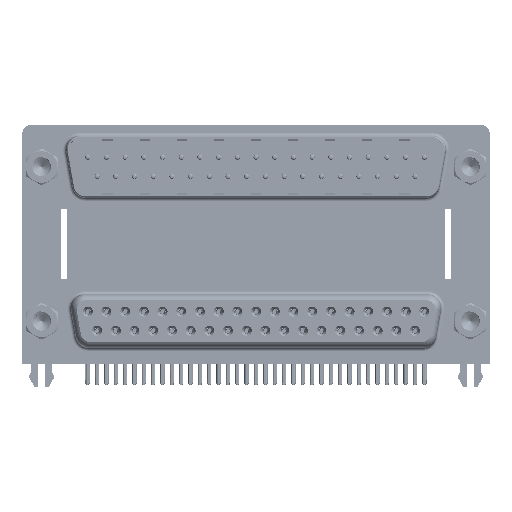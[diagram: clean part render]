
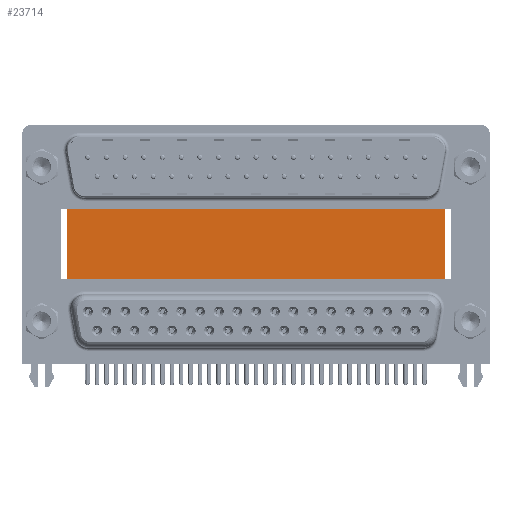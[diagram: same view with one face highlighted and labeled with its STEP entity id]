
A CAD part, top view. The second image highlights one B-rep face of the part: STEP entity #23714.
In plain terms, the highlighted planar face has unit normal (0, 0, 1).
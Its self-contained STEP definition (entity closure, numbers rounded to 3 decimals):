
#1918 = EDGE_CURVE ( 'NONE', #43277, #64732, #73841, .T. ) ;
#3527 = CARTESIAN_POINT ( 'NONE',  ( 3.79, 16.585, -12. ) ) ;
#3549 = CARTESIAN_POINT ( 'NONE',  ( 59.71, 16.585, -12. ) ) ;
#8940 = VERTEX_POINT ( 'NONE', #35187 ) ;
#10958 = ORIENTED_EDGE ( 'NONE', *, *, #48149, .F. ) ;
#12147 = ORIENTED_EDGE ( 'NONE', *, *, #1918, .F. ) ;
#13988 = LINE ( 'NONE', #25743, #72614 ) ;
#17152 = CARTESIAN_POINT ( 'NONE',  ( 59.71, 16.585, -12. ) ) ;
#21014 = DIRECTION ( 'NONE',  ( -1., 0., 0. ) ) ;
#23714 = ADVANCED_FACE ( 'NONE', ( #49443 ), #66976, .F. ) ;
#24715 = CARTESIAN_POINT ( 'NONE',  ( 3.79, -3.735, -12. ) ) ;
#25743 = CARTESIAN_POINT ( 'NONE',  ( 3.79, 16.585, -12. ) ) ;
#26696 = DIRECTION ( 'NONE',  ( 0., 0., -1. ) ) ;
#26873 = CARTESIAN_POINT ( 'NONE',  ( 59.71, -3.735, -12. ) ) ;
#29584 = EDGE_LOOP ( 'NONE', ( #45583, #12147, #10958, #63220 ) ) ;
#30680 = DIRECTION ( 'NONE',  ( 0., -1., 0. ) ) ;
#31212 = CARTESIAN_POINT ( 'NONE',  ( 3.79, 16.585, -12. ) ) ;
#34984 = VECTOR ( 'NONE', #59253, 1000. ) ;
#35187 = CARTESIAN_POINT ( 'NONE',  ( 3.79, 16.585, -12. ) ) ;
#35402 = LINE ( 'NONE', #31212, #56946 ) ;
#40063 = VERTEX_POINT ( 'NONE', #56469 ) ;
#43277 = VERTEX_POINT ( 'NONE', #17152 ) ;
#45583 = ORIENTED_EDGE ( 'NONE', *, *, #53203, .T. ) ;
#48149 = EDGE_CURVE ( 'NONE', #8940, #43277, #35402, .T. ) ;
#49443 = FACE_OUTER_BOUND ( 'NONE', #29584, .T. ) ;
#53203 = EDGE_CURVE ( 'NONE', #40063, #64732, #69924, .T. ) ;
#55121 = DIRECTION ( 'NONE',  ( 1., 0., 0. ) ) ;
#56469 = CARTESIAN_POINT ( 'NONE',  ( 3.79, -3.735, -12. ) ) ;
#56946 = VECTOR ( 'NONE', #55121, 1000. ) ;
#59253 = DIRECTION ( 'NONE',  ( 1., 0., 0. ) ) ;
#60428 = AXIS2_PLACEMENT_3D ( 'NONE', #3527, #26696, #21014 ) ;
#63220 = ORIENTED_EDGE ( 'NONE', *, *, #74331, .T. ) ;
#64130 = VECTOR ( 'NONE', #74212, 1000. ) ;
#64732 = VERTEX_POINT ( 'NONE', #26873 ) ;
#66976 = PLANE ( 'NONE',  #60428 ) ;
#69924 = LINE ( 'NONE', #24715, #34984 ) ;
#72614 = VECTOR ( 'NONE', #30680, 1000. ) ;
#73841 = LINE ( 'NONE', #3549, #64130 ) ;
#74212 = DIRECTION ( 'NONE',  ( 0., -1., 0. ) ) ;
#74331 = EDGE_CURVE ( 'NONE', #8940, #40063, #13988, .T. ) ;
